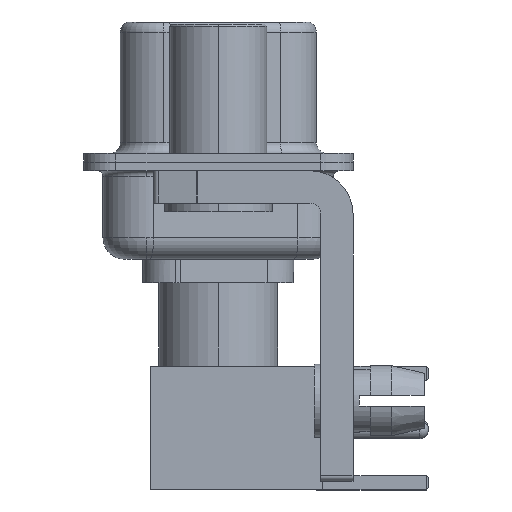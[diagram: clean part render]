
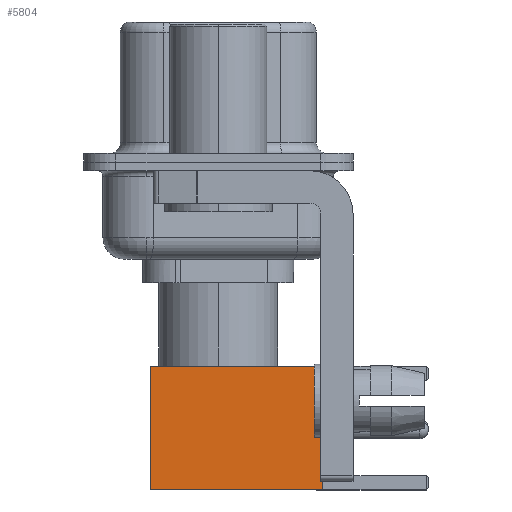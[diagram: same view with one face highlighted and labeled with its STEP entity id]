
A CAD part, left-side view. The second image highlights one B-rep face of the part: STEP entity #5804.
In plain terms, the highlighted face is planar.
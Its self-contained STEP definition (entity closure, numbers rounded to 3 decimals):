
#230 = ORIENTED_EDGE ( 'NONE', *, *, #3224, .F. ) ;
#1168 = VECTOR ( 'NONE', #12492, 1000. ) ;
#1423 = DIRECTION ( 'NONE',  ( 0., 0., 1. ) ) ;
#1781 = EDGE_CURVE ( 'NONE', #12817, #12757, #5978, .T. ) ;
#1852 = ORIENTED_EDGE ( 'NONE', *, *, #5512, .T. ) ;
#2450 = VERTEX_POINT ( 'NONE', #11661 ) ;
#2819 = DIRECTION ( 'NONE',  ( 0., 1., 0. ) ) ;
#3224 = EDGE_CURVE ( 'NONE', #17939, #12757, #4112, .T. ) ;
#3286 = FACE_OUTER_BOUND ( 'NONE', #16803, .T. ) ;
#3641 = LINE ( 'NONE', #16226, #1168 ) ;
#4112 = LINE ( 'NONE', #9231, #16829 ) ;
#5512 = EDGE_CURVE ( 'NONE', #2450, #12817, #3641, .T. ) ;
#5724 = CARTESIAN_POINT ( 'NONE',  ( -2.875, 2.875, 0. ) ) ;
#5804 = ADVANCED_FACE ( 'NONE', ( #3286 ), #21027, .T. ) ;
#5978 = LINE ( 'NONE', #21619, #7301 ) ;
#7301 = VECTOR ( 'NONE', #21858, 1000. ) ;
#8289 = DIRECTION ( 'NONE',  ( -1., 0., 0. ) ) ;
#8602 = AXIS2_PLACEMENT_3D ( 'NONE', #22643, #2819, #1423 ) ;
#8707 = VECTOR ( 'NONE', #8289, 1000. ) ;
#9231 = CARTESIAN_POINT ( 'NONE',  ( -2.875, 2.875, 0. ) ) ;
#10381 = CARTESIAN_POINT ( 'NONE',  ( 0., 2.875, 8. ) ) ;
#11661 = CARTESIAN_POINT ( 'NONE',  ( 2.875, 2.875, 8. ) ) ;
#12492 = DIRECTION ( 'NONE',  ( 0., 0., -1. ) ) ;
#12757 = VERTEX_POINT ( 'NONE', #5724 ) ;
#12817 = VERTEX_POINT ( 'NONE', #21378 ) ;
#13118 = ORIENTED_EDGE ( 'NONE', *, *, #1781, .T. ) ;
#16226 = CARTESIAN_POINT ( 'NONE',  ( 2.875, 2.875, 0. ) ) ;
#16480 = DIRECTION ( 'NONE',  ( 0., 0., -1. ) ) ;
#16803 = EDGE_LOOP ( 'NONE', ( #1852, #13118, #230, #19577 ) ) ;
#16829 = VECTOR ( 'NONE', #16480, 1000. ) ;
#17903 = EDGE_CURVE ( 'NONE', #2450, #17939, #19146, .T. ) ;
#17939 = VERTEX_POINT ( 'NONE', #22874 ) ;
#19146 = LINE ( 'NONE', #10381, #8707 ) ;
#19577 = ORIENTED_EDGE ( 'NONE', *, *, #17903, .F. ) ;
#21027 = PLANE ( 'NONE',  #8602 ) ;
#21378 = CARTESIAN_POINT ( 'NONE',  ( 2.875, 2.875, 0. ) ) ;
#21619 = CARTESIAN_POINT ( 'NONE',  ( 0., 2.875, 0. ) ) ;
#21858 = DIRECTION ( 'NONE',  ( -1., 0., 0. ) ) ;
#22643 = CARTESIAN_POINT ( 'NONE',  ( 2.875, 2.875, 0. ) ) ;
#22874 = CARTESIAN_POINT ( 'NONE',  ( -2.875, 2.875, 8. ) ) ;
